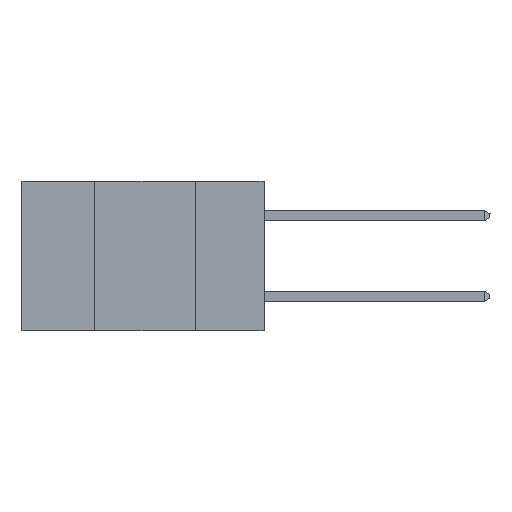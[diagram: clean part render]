
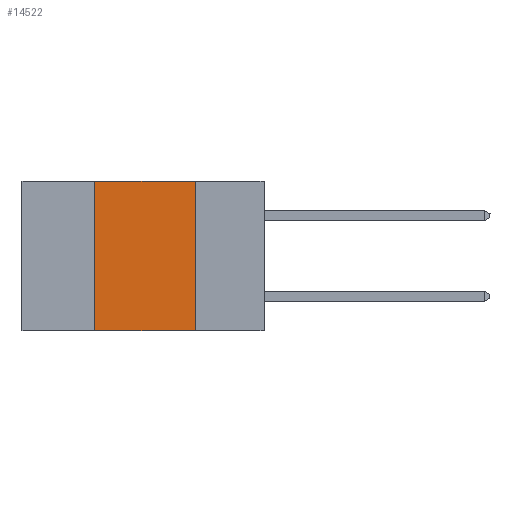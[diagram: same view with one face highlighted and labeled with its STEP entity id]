
A CAD part, left-side view. The second image highlights one B-rep face of the part: STEP entity #14522.
In plain terms, the highlighted planar face has unit normal (-1, 0, 0).
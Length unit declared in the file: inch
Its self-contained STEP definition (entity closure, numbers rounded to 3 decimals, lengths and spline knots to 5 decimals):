
#288 = CARTESIAN_POINT ( 'NONE',  ( 0., 0.6, 0. ) ) ;
#601 = LINE ( 'NONE', #14919, #4756 ) ;
#918 = CARTESIAN_POINT ( 'NONE',  ( 0., 0.17, -0.37 ) ) ;
#2059 = DIRECTION ( 'NONE',  ( 1., 0., 0. ) ) ;
#2612 = DIRECTION ( 'NONE',  ( 0., -1., 0. ) ) ;
#3025 = CARTESIAN_POINT ( 'NONE',  ( 0., 0.42, -0.37 ) ) ;
#3270 = VERTEX_POINT ( 'NONE', #7110 ) ;
#3396 = VECTOR ( 'NONE', #2612, 39.37008 ) ;
#3570 = CARTESIAN_POINT ( 'NONE',  ( 0., 0.17, 0. ) ) ;
#3802 = EDGE_CURVE ( 'NONE', #3270, #7807, #18278, .T. ) ;
#4252 = DIRECTION ( 'NONE',  ( 0., 0., 1. ) ) ;
#4756 = VECTOR ( 'NONE', #4252, 39.37008 ) ;
#5039 = AXIS2_PLACEMENT_3D ( 'NONE', #12430, #2059, #7174 ) ;
#6625 = EDGE_CURVE ( 'NONE', #14689, #17190, #13478, .T. ) ;
#6682 = EDGE_CURVE ( 'NONE', #14689, #3270, #601, .T. ) ;
#7110 = CARTESIAN_POINT ( 'NONE',  ( 0., 0.42, 0. ) ) ;
#7174 = DIRECTION ( 'NONE',  ( 0., 0., -1. ) ) ;
#7807 = VERTEX_POINT ( 'NONE', #10018 ) ;
#10018 = CARTESIAN_POINT ( 'NONE',  ( 0., 0.17, 0. ) ) ;
#10292 = LINE ( 'NONE', #3570, #12849 ) ;
#10668 = DIRECTION ( 'NONE',  ( 0., 0., -1. ) ) ;
#12430 = CARTESIAN_POINT ( 'NONE',  ( 0., 0.6, 0. ) ) ;
#12849 = VECTOR ( 'NONE', #10668, 39.37008 ) ;
#12987 = FACE_OUTER_BOUND ( 'NONE', #18238, .T. ) ;
#13478 = LINE ( 'NONE', #20424, #3396 ) ;
#13807 = ORIENTED_EDGE ( 'NONE', *, *, #6682, .F. ) ;
#14522 = ADVANCED_FACE ( 'NONE', ( #12987 ), #23032, .F. ) ;
#14689 = VERTEX_POINT ( 'NONE', #3025 ) ;
#14919 = CARTESIAN_POINT ( 'NONE',  ( 0., 0.42, 0. ) ) ;
#16243 = DIRECTION ( 'NONE',  ( 0., -1., 0. ) ) ;
#17190 = VERTEX_POINT ( 'NONE', #918 ) ;
#18010 = ORIENTED_EDGE ( 'NONE', *, *, #3802, .F. ) ;
#18238 = EDGE_LOOP ( 'NONE', ( #22153, #18010, #13807, #20259 ) ) ;
#18278 = LINE ( 'NONE', #288, #21013 ) ;
#18407 = EDGE_CURVE ( 'NONE', #7807, #17190, #10292, .T. ) ;
#20259 = ORIENTED_EDGE ( 'NONE', *, *, #6625, .T. ) ;
#20424 = CARTESIAN_POINT ( 'NONE',  ( 0., 0.6, -0.37 ) ) ;
#21013 = VECTOR ( 'NONE', #16243, 39.37008 ) ;
#22153 = ORIENTED_EDGE ( 'NONE', *, *, #18407, .F. ) ;
#23032 = PLANE ( 'NONE',  #5039 ) ;
